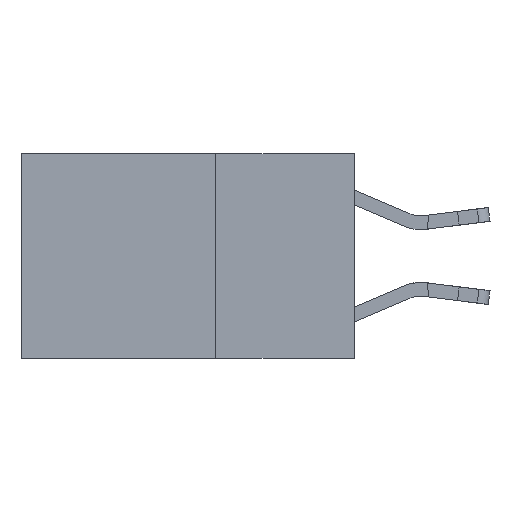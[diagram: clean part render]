
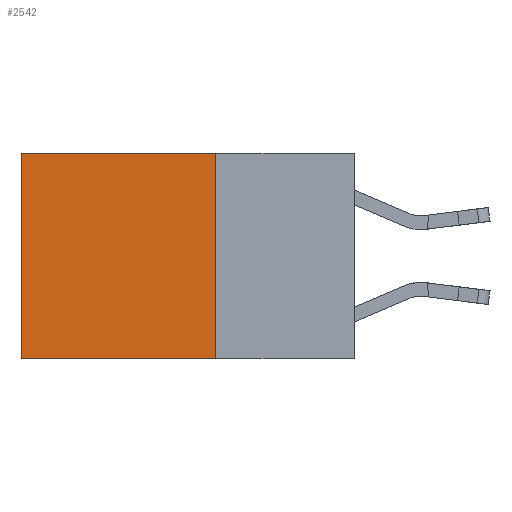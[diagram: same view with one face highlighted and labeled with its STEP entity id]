
A CAD part, left-side view. The second image highlights one B-rep face of the part: STEP entity #2542.
In plain terms, the highlighted planar face has unit normal (-1, 0, 0).
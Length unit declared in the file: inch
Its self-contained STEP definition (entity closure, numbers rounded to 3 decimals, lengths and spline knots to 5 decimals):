
#650 = ORIENTED_EDGE ( 'NONE', *, *, #18565, .T. ) ;
#775 = ORIENTED_EDGE ( 'NONE', *, *, #19303, .T. ) ;
#2369 = ORIENTED_EDGE ( 'NONE', *, *, #8696, .F. ) ;
#2542 = ADVANCED_FACE ( 'NONE', ( #17016 ), #5306, .F. ) ;
#2566 = LINE ( 'NONE', #11286, #11875 ) ;
#3065 = DIRECTION ( 'NONE',  ( 0., 0., -1. ) ) ;
#4016 = DIRECTION ( 'NONE',  ( 0., 1., 0. ) ) ;
#5155 = EDGE_CURVE ( 'NONE', #5998, #15680, #2566, .T. ) ;
#5306 = PLANE ( 'NONE',  #7761 ) ;
#5490 = LINE ( 'NONE', #7138, #14741 ) ;
#5998 = VERTEX_POINT ( 'NONE', #14198 ) ;
#7138 = CARTESIAN_POINT ( 'NONE',  ( 0.2625, 0.6, 0. ) ) ;
#7761 = AXIS2_PLACEMENT_3D ( 'NONE', #15723, #11289, #18127 ) ;
#8173 = VECTOR ( 'NONE', #8782, 39.37008 ) ;
#8696 = EDGE_CURVE ( 'NONE', #10188, #5998, #10488, .T. ) ;
#8782 = DIRECTION ( 'NONE',  ( 0., 1., 0. ) ) ;
#8840 = VECTOR ( 'NONE', #3065, 39.37008 ) ;
#9043 = VERTEX_POINT ( 'NONE', #13333 ) ;
#10188 = VERTEX_POINT ( 'NONE', #10620 ) ;
#10413 = CARTESIAN_POINT ( 'NONE',  ( 0.2625, 0.6, -0.37 ) ) ;
#10488 = LINE ( 'NONE', #16613, #8840 ) ;
#10620 = CARTESIAN_POINT ( 'NONE',  ( 0.2625, 0.25, 0. ) ) ;
#11286 = CARTESIAN_POINT ( 'NONE',  ( 0.2625, 0.25, -0.37 ) ) ;
#11289 = DIRECTION ( 'NONE',  ( 1., 0., 0. ) ) ;
#11875 = VECTOR ( 'NONE', #4016, 39.37008 ) ;
#13333 = CARTESIAN_POINT ( 'NONE',  ( 0.2625, 0.6, 0. ) ) ;
#14198 = CARTESIAN_POINT ( 'NONE',  ( 0.2625, 0.25, -0.37 ) ) ;
#14698 = DIRECTION ( 'NONE',  ( 0., 0., -1. ) ) ;
#14741 = VECTOR ( 'NONE', #14698, 39.37008 ) ;
#15680 = VERTEX_POINT ( 'NONE', #10413 ) ;
#15723 = CARTESIAN_POINT ( 'NONE',  ( 0.2625, 0.25, 0. ) ) ;
#16260 = CARTESIAN_POINT ( 'NONE',  ( 0.2625, 0.25, 0. ) ) ;
#16613 = CARTESIAN_POINT ( 'NONE',  ( 0.2625, 0.25, 0. ) ) ;
#17016 = FACE_OUTER_BOUND ( 'NONE', #17970, .T. ) ;
#17970 = EDGE_LOOP ( 'NONE', ( #650, #18635, #2369, #775 ) ) ;
#18127 = DIRECTION ( 'NONE',  ( 0., 0., -1. ) ) ;
#18227 = LINE ( 'NONE', #16260, #8173 ) ;
#18565 = EDGE_CURVE ( 'NONE', #9043, #15680, #5490, .T. ) ;
#18635 = ORIENTED_EDGE ( 'NONE', *, *, #5155, .F. ) ;
#19303 = EDGE_CURVE ( 'NONE', #10188, #9043, #18227, .T. ) ;
